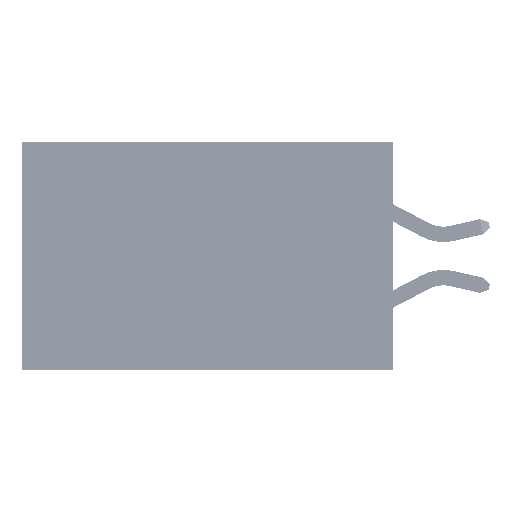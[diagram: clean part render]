
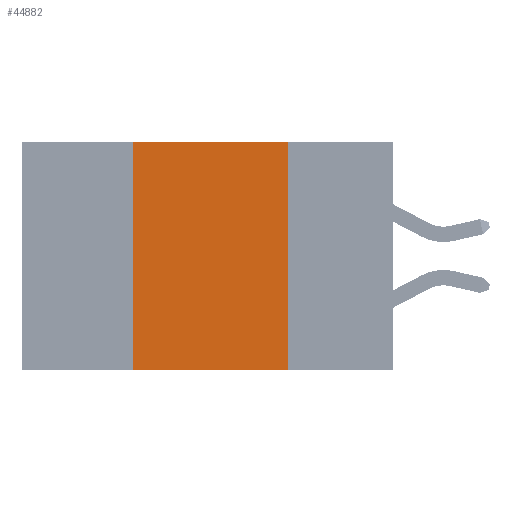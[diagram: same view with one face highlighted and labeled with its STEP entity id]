
A CAD part, left-side view. The second image highlights one B-rep face of the part: STEP entity #44882.
In plain terms, the highlighted planar face has unit normal (-1, 0, 0).
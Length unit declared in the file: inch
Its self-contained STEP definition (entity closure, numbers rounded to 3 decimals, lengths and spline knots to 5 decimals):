
#481 = DIRECTION ( 'NONE',  ( 0., -1., 0. ) ) ;
#499 = VECTOR ( 'NONE', #481, 39.37008 ) ;
#1270 = EDGE_CURVE ( 'NONE', #33807, #36833, #44026, .T. ) ;
#3759 = VECTOR ( 'NONE', #9505, 39.37008 ) ;
#4659 = LINE ( 'NONE', #16968, #27988 ) ;
#4851 = DIRECTION ( 'NONE',  ( 1., 0., 0. ) ) ;
#5485 = FACE_OUTER_BOUND ( 'NONE', #23141, .T. ) ;
#6771 = VERTEX_POINT ( 'NONE', #37592 ) ;
#8458 = CARTESIAN_POINT ( 'NONE',  ( 0., 0.6, 0. ) ) ;
#9505 = DIRECTION ( 'NONE',  ( 0., -1., 0. ) ) ;
#10790 = CARTESIAN_POINT ( 'NONE',  ( 0., 0.6, -0.37 ) ) ;
#15385 = DIRECTION ( 'NONE',  ( 0., 0., -1. ) ) ;
#16406 = CARTESIAN_POINT ( 'NONE',  ( 0., 0.42, 0. ) ) ;
#16968 = CARTESIAN_POINT ( 'NONE',  ( 0., 0.42, 0. ) ) ;
#17868 = LINE ( 'NONE', #10790, #499 ) ;
#18209 = EDGE_CURVE ( 'NONE', #36833, #19709, #24050, .T. ) ;
#18764 = DIRECTION ( 'NONE',  ( 0., 0., -1. ) ) ;
#19355 = AXIS2_PLACEMENT_3D ( 'NONE', #8458, #4851, #18764 ) ;
#19709 = VERTEX_POINT ( 'NONE', #32916 ) ;
#20545 = ORIENTED_EDGE ( 'NONE', *, *, #18209, .F. ) ;
#22988 = ORIENTED_EDGE ( 'NONE', *, *, #42953, .T. ) ;
#23141 = EDGE_LOOP ( 'NONE', ( #20545, #33853, #39504, #22988 ) ) ;
#23633 = DIRECTION ( 'NONE',  ( 0., 0., 1. ) ) ;
#24050 = LINE ( 'NONE', #35591, #39310 ) ;
#25607 = PLANE ( 'NONE',  #19355 ) ;
#27988 = VECTOR ( 'NONE', #23633, 39.37008 ) ;
#30974 = CARTESIAN_POINT ( 'NONE',  ( 0., 0.6, 0. ) ) ;
#32916 = CARTESIAN_POINT ( 'NONE',  ( 0., 0.17, -0.37 ) ) ;
#33807 = VERTEX_POINT ( 'NONE', #16406 ) ;
#33853 = ORIENTED_EDGE ( 'NONE', *, *, #1270, .F. ) ;
#35591 = CARTESIAN_POINT ( 'NONE',  ( 0., 0.17, 0. ) ) ;
#36833 = VERTEX_POINT ( 'NONE', #39581 ) ;
#37592 = CARTESIAN_POINT ( 'NONE',  ( 0., 0.42, -0.37 ) ) ;
#38881 = EDGE_CURVE ( 'NONE', #6771, #33807, #4659, .T. ) ;
#39310 = VECTOR ( 'NONE', #15385, 39.37008 ) ;
#39504 = ORIENTED_EDGE ( 'NONE', *, *, #38881, .F. ) ;
#39581 = CARTESIAN_POINT ( 'NONE',  ( 0., 0.17, 0. ) ) ;
#42953 = EDGE_CURVE ( 'NONE', #6771, #19709, #17868, .T. ) ;
#44026 = LINE ( 'NONE', #30974, #3759 ) ;
#44882 = ADVANCED_FACE ( 'NONE', ( #5485 ), #25607, .F. ) ;
